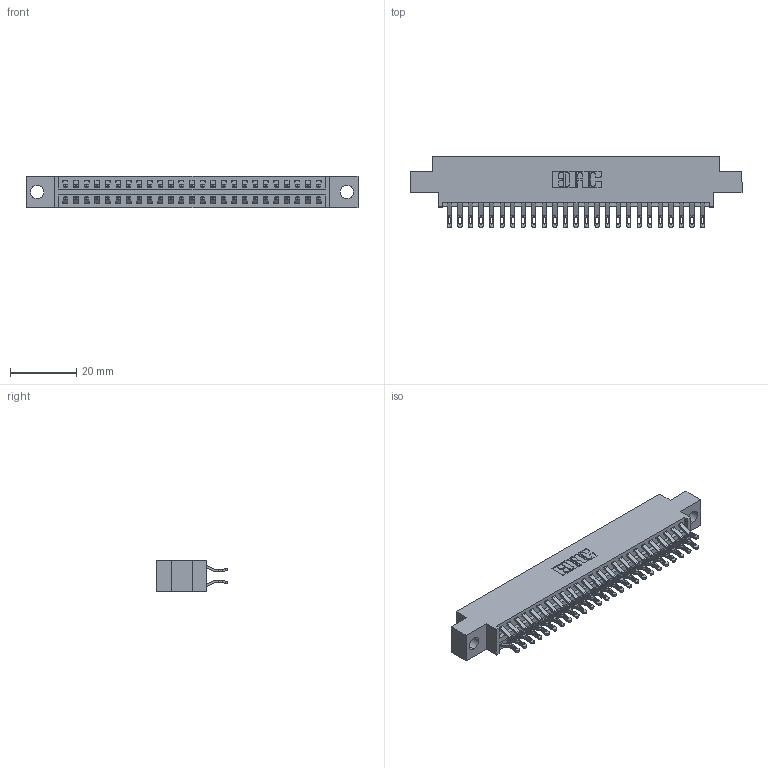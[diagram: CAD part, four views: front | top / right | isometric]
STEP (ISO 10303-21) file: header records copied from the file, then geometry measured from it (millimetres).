
FILE_DESCRIPTION (( 'STEP AP203' ), '1' );
FILE_NAME ('346-050-555-804.STEP', '2022-05-20T23:39:42', ( '' ), ( '' ), 'SwSTEP 2.0', 'SolidWorks 2020', '' );
FILE_SCHEMA (( 'CONFIG_CONTROL_DESIGN' ));
Length unit declared in the file: inch
Products named in the file (3): 345-292-001_555 Tail; 346-050-555-804; 346 Part_0.170 Offset - 0.156 Dia-TH
Assembly tree (51 placements, depth 2):
  346-050-555-804
    346 Part_0.170 Offset - 0.156 Dia-TH
    345-292-001_555 Tail  x50
Bounding box: 99.95 x 21.46 x 9.4 mm (x, y, z)
Volume: 9498.7 mm3; surface area: 13333.9 mm2
Topology: 51 solids, 51 shells, 3040 faces, 9527 edges, 6350 vertices
Faces by surface type: plane 1744, cylinder 1296
Entity records: 19481 total; most frequent: CARTESIAN_POINT 3276, ORIENTED_EDGE 3178, DIRECTION 2905, EDGE_CURVE 1589, LINE 1337, VECTOR 1337, VERTEX_POINT 1058, AXIS2_PLACEMENT_3D 784
